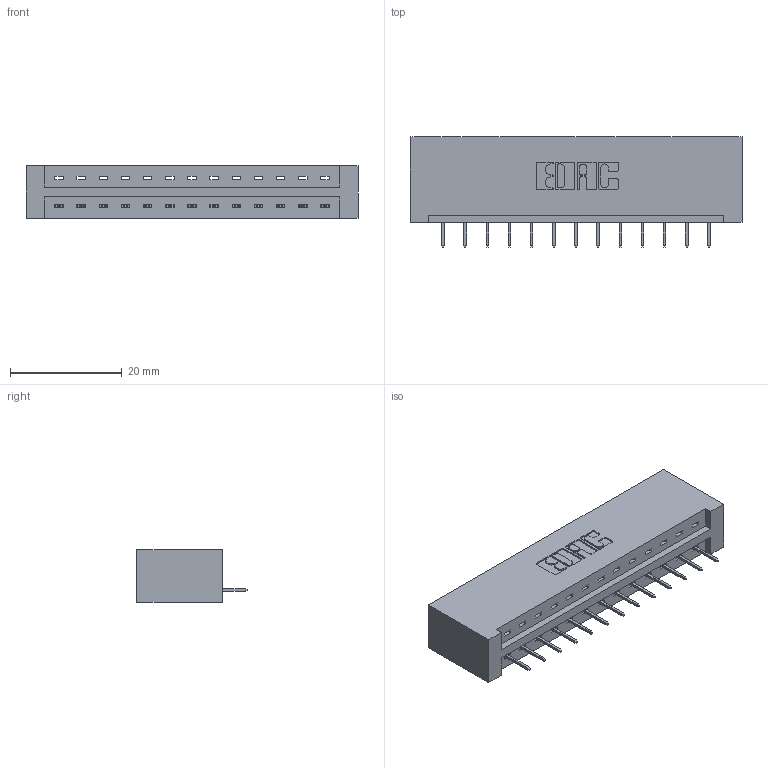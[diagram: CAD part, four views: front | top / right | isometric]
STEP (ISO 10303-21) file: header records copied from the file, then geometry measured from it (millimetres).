
FILE_DESCRIPTION (( 'STEP AP203' ), '1' );
FILE_NAME ('337-013-524-101.STEP', '2019-09-28T01:46:32', ( '' ), ( '' ), 'SwSTEP 2.0', 'SolidWorks 2016', '' );
FILE_SCHEMA (( 'CONFIG_CONTROL_DESIGN' ));
Length unit declared in the file: inch
Products named in the file (3): 337-013-524-101; 337 Part_No Mounting Lugs; 345-292-001_345-293-124
Assembly tree (14 placements, depth 2):
  337-013-524-101
    337 Part_No Mounting Lugs
    345-292-001_345-293-124  x13
Bounding box: 59.39 x 19.69 x 9.4 mm (x, y, z)
Volume: 6496.6 mm3; surface area: 6353.1 mm2
Topology: 14 solids, 14 shells, 964 faces, 2783 edges, 1802 vertices
Faces by surface type: plane 742, cylinder 222
Entity records: 13211 total; most frequent: CARTESIAN_POINT 2305, ORIENTED_EDGE 2254, DIRECTION 1993, EDGE_CURVE 1127, VECTOR 1011, LINE 1011, VERTEX_POINT 746, AXIS2_PLACEMENT_3D 491
